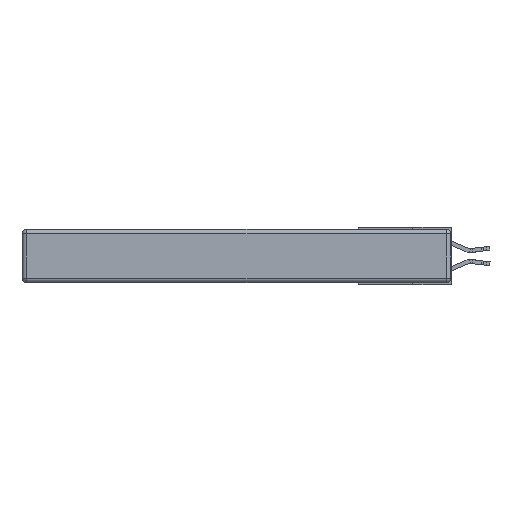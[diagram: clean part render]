
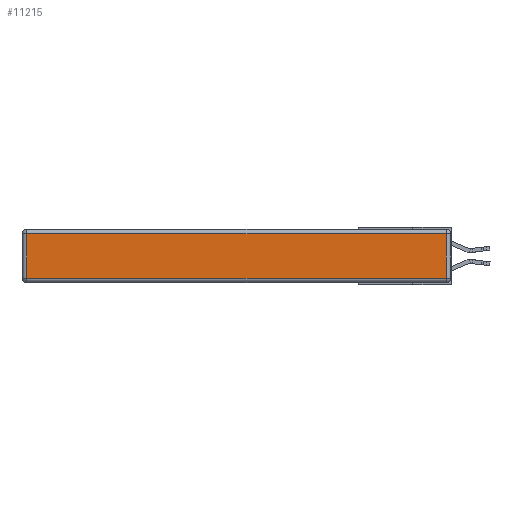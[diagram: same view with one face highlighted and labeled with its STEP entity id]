
A CAD part, left-side view. The second image highlights one B-rep face of the part: STEP entity #11215.
In plain terms, the highlighted planar face has unit normal (-1, 0, 0).
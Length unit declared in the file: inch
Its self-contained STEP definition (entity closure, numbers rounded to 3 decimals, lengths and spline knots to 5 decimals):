
#668 = CARTESIAN_POINT ( 'NONE',  ( 0., 0., -0.313 ) ) ;
#3283 = ORIENTED_EDGE ( 'NONE', *, *, #25629, .T. ) ;
#3916 = AXIS2_PLACEMENT_3D ( 'NONE', #26996, #24632, #27105 ) ;
#4057 = VERTEX_POINT ( 'NONE', #17685 ) ;
#5215 = EDGE_CURVE ( 'NONE', #4057, #16434, #22636, .T. ) ;
#5662 = LINE ( 'NONE', #26163, #18229 ) ;
#6712 = VECTOR ( 'NONE', #30779, 39.37008 ) ;
#11215 = ADVANCED_FACE ( 'NONE', ( #13741 ), #12315, .T. ) ;
#12315 = PLANE ( 'NONE',  #3916 ) ;
#12645 = DIRECTION ( 'NONE',  ( 0., 0., -1. ) ) ;
#13097 = DIRECTION ( 'NONE',  ( 0., 0., 1. ) ) ;
#13741 = FACE_OUTER_BOUND ( 'NONE', #27786, .T. ) ;
#13924 = CARTESIAN_POINT ( 'NONE',  ( 0., 2.72, -0.313 ) ) ;
#14862 = ORIENTED_EDGE ( 'NONE', *, *, #5215, .T. ) ;
#15172 = EDGE_CURVE ( 'NONE', #24690, #4057, #26437, .T. ) ;
#15532 = VERTEX_POINT ( 'NONE', #26089 ) ;
#16157 = LINE ( 'NONE', #668, #6712 ) ;
#16434 = VERTEX_POINT ( 'NONE', #13924 ) ;
#17685 = CARTESIAN_POINT ( 'NONE',  ( 0., 2.72, -0.03 ) ) ;
#18229 = VECTOR ( 'NONE', #13097, 39.37008 ) ;
#19175 = CARTESIAN_POINT ( 'NONE',  ( 0., 2.75, -0.03 ) ) ;
#19681 = CARTESIAN_POINT ( 'NONE',  ( 0., 2.72, -0.343 ) ) ;
#20617 = ORIENTED_EDGE ( 'NONE', *, *, #27618, .T. ) ;
#22636 = LINE ( 'NONE', #19681, #29278 ) ;
#24632 = DIRECTION ( 'NONE',  ( -1., 0., 0. ) ) ;
#24690 = VERTEX_POINT ( 'NONE', #24758 ) ;
#24758 = CARTESIAN_POINT ( 'NONE',  ( 0., 0.03, -0.03 ) ) ;
#25629 = EDGE_CURVE ( 'NONE', #15532, #24690, #5662, .T. ) ;
#25656 = VECTOR ( 'NONE', #26950, 39.37008 ) ;
#26089 = CARTESIAN_POINT ( 'NONE',  ( 0., 0.03, -0.313 ) ) ;
#26163 = CARTESIAN_POINT ( 'NONE',  ( 0., 0.03, -0.343 ) ) ;
#26437 = LINE ( 'NONE', #19175, #25656 ) ;
#26950 = DIRECTION ( 'NONE',  ( 0., 1., 0. ) ) ;
#26996 = CARTESIAN_POINT ( 'NONE',  ( 0., 0., -0.343 ) ) ;
#27105 = DIRECTION ( 'NONE',  ( 0., 0., 1. ) ) ;
#27618 = EDGE_CURVE ( 'NONE', #16434, #15532, #16157, .T. ) ;
#27786 = EDGE_LOOP ( 'NONE', ( #20617, #3283, #27851, #14862 ) ) ;
#27851 = ORIENTED_EDGE ( 'NONE', *, *, #15172, .T. ) ;
#29278 = VECTOR ( 'NONE', #12645, 39.37008 ) ;
#30779 = DIRECTION ( 'NONE',  ( 0., -1., 0. ) ) ;
